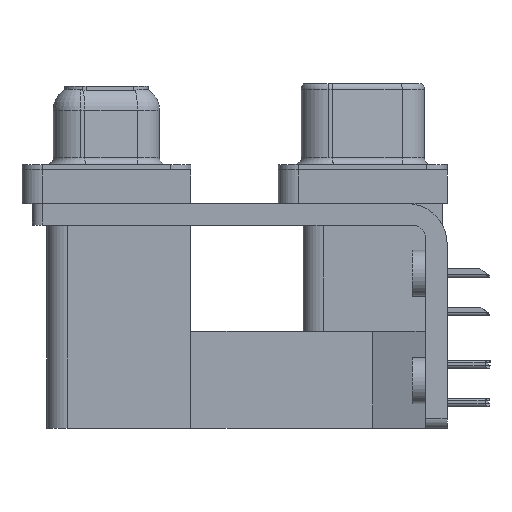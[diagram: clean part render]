
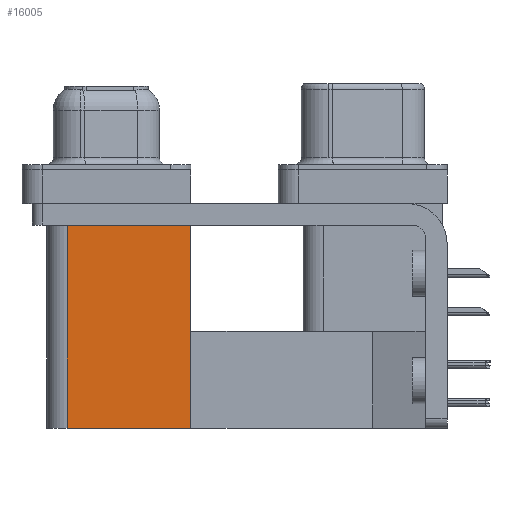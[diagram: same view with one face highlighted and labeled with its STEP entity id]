
A CAD part, left-side view. The second image highlights one B-rep face of the part: STEP entity #16005.
In plain terms, the highlighted planar face has unit normal (-1, 0, 0).
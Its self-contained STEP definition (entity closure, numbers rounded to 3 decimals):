
#436 = VERTEX_POINT ( 'NONE', #26334 ) ;
#3341 = LINE ( 'NONE', #5564, #8746 ) ;
#4583 = ORIENTED_EDGE ( 'NONE', *, *, #23501, .F. ) ;
#4715 = EDGE_CURVE ( 'NONE', #13212, #436, #3341, .T. ) ;
#5564 = CARTESIAN_POINT ( 'NONE',  ( 3.79, 12.775, -19.2 ) ) ;
#6006 = LINE ( 'NONE', #15829, #35515 ) ;
#8267 = DIRECTION ( 'NONE',  ( 0., 0., 1. ) ) ;
#8746 = VECTOR ( 'NONE', #30452, 1000. ) ;
#9417 = DIRECTION ( 'NONE',  ( 0., 1., 0. ) ) ;
#9819 = VERTEX_POINT ( 'NONE', #24415 ) ;
#12957 = FACE_OUTER_BOUND ( 'NONE', #29540, .T. ) ;
#13212 = VERTEX_POINT ( 'NONE', #17824 ) ;
#13963 = VERTEX_POINT ( 'NONE', #21676 ) ;
#15829 = CARTESIAN_POINT ( 'NONE',  ( 3.79, 12.775, -2.5 ) ) ;
#16005 = ADVANCED_FACE ( 'NONE', ( #12957 ), #25394, .F. ) ;
#16555 = ORIENTED_EDGE ( 'NONE', *, *, #25896, .F. ) ;
#17824 = CARTESIAN_POINT ( 'NONE',  ( 3.79, 12.775, -19.2 ) ) ;
#19813 = ORIENTED_EDGE ( 'NONE', *, *, #25160, .T. ) ;
#20057 = VECTOR ( 'NONE', #34740, 1000. ) ;
#21676 = CARTESIAN_POINT ( 'NONE',  ( 3.79, 21.975, -2.5 ) ) ;
#22367 = CARTESIAN_POINT ( 'NONE',  ( 3.79, 12.775, -19.2 ) ) ;
#23501 = EDGE_CURVE ( 'NONE', #13212, #9819, #34329, .T. ) ;
#23718 = CARTESIAN_POINT ( 'NONE',  ( 3.79, 21.975, -19.2 ) ) ;
#23954 = DIRECTION ( 'NONE',  ( 1., 0., 0. ) ) ;
#24268 = ORIENTED_EDGE ( 'NONE', *, *, #4715, .T. ) ;
#24415 = CARTESIAN_POINT ( 'NONE',  ( 3.79, 21.975, -19.2 ) ) ;
#24912 = CARTESIAN_POINT ( 'NONE',  ( 3.79, 12.775, -19.2 ) ) ;
#25160 = EDGE_CURVE ( 'NONE', #436, #13963, #6006, .T. ) ;
#25394 = PLANE ( 'NONE',  #37995 ) ;
#25896 = EDGE_CURVE ( 'NONE', #9819, #13963, #29164, .T. ) ;
#26334 = CARTESIAN_POINT ( 'NONE',  ( 3.79, 12.775, -2.5 ) ) ;
#29164 = LINE ( 'NONE', #23718, #33536 ) ;
#29540 = EDGE_LOOP ( 'NONE', ( #19813, #16555, #4583, #24268 ) ) ;
#30452 = DIRECTION ( 'NONE',  ( 0., 0., 1. ) ) ;
#32986 = DIRECTION ( 'NONE',  ( 0., 1., 0. ) ) ;
#33536 = VECTOR ( 'NONE', #8267, 1000. ) ;
#34329 = LINE ( 'NONE', #24912, #20057 ) ;
#34740 = DIRECTION ( 'NONE',  ( 0., 1., 0. ) ) ;
#35515 = VECTOR ( 'NONE', #9417, 1000. ) ;
#37995 = AXIS2_PLACEMENT_3D ( 'NONE', #22367, #23954, #32986 ) ;
